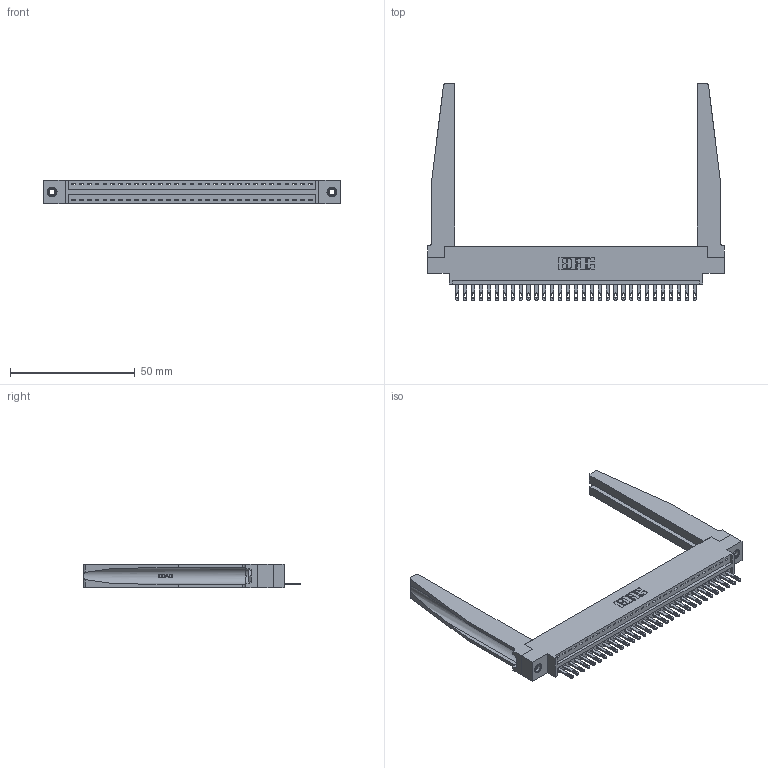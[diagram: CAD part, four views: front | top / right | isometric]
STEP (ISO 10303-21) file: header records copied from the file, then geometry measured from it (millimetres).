
FILE_DESCRIPTION (( 'STEP AP203' ), '1' );
FILE_NAME ('346-031-500-678.STEP', '2022-05-06T16:28:09', ( '' ), ( '' ), 'SwSTEP 2.0', 'SolidWorks 2020', '' );
FILE_SCHEMA (( 'CONFIG_CONTROL_DESIGN' ));
Length unit declared in the file: inch
Products named in the file (5): 346 Part_0.170 Offset - 0.156 Dia-TH; 346-031-500-678; 345-292-001_345-293-100; 346-220-078_345-220-078; 345-250-001_345-250-001-102
Assembly tree (36 placements, depth 2):
  346-031-500-678
    346 Part_0.170 Offset - 0.156 Dia-TH
    345-292-001_345-293-100  x31
    346-220-078_345-220-078  x2
    345-250-001_345-250-001-102  x2
Bounding box: 119 x 87.12 x 9.4 mm (x, y, z)
Volume: 18070.4 mm3; surface area: 20636.7 mm2
Topology: 36 solids, 36 shells, 2048 faces, 6193 edges, 4118 vertices
Faces by surface type: plane 1290, cylinder 706, bspline 36, cone 12, torus 4
Entity records: 25946 total; most frequent: CARTESIAN_POINT 5366, ORIENTED_EDGE 4218, DIRECTION 3733, EDGE_CURVE 2109, LINE 1755, VECTOR 1755, VERTEX_POINT 1400, AXIS2_PLACEMENT_3D 989
